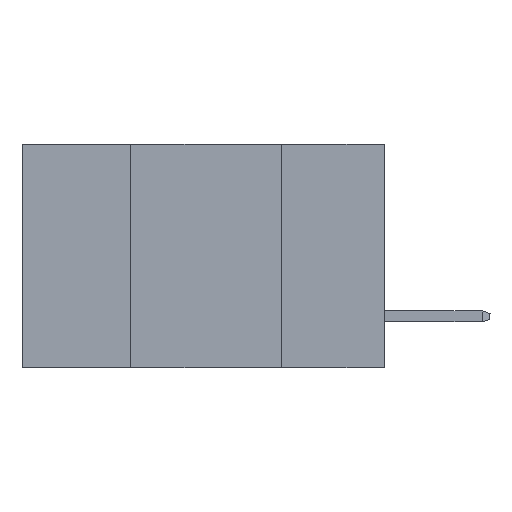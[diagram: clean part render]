
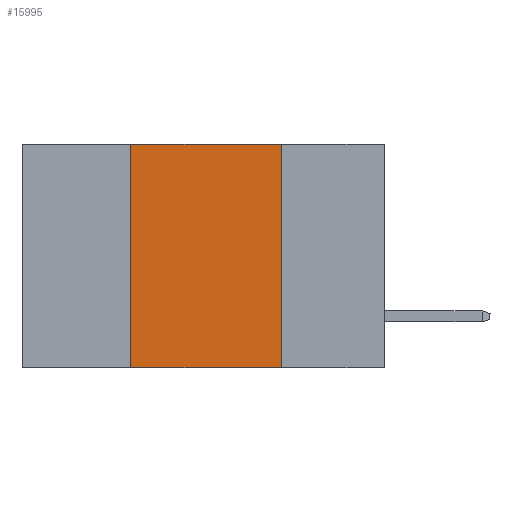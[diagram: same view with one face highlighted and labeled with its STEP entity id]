
A CAD part, left-side view. The second image highlights one B-rep face of the part: STEP entity #15995.
In plain terms, the highlighted planar face has unit normal (-1, 0, 0).
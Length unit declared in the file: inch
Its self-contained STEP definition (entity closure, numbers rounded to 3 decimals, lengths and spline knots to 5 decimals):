
#517 = CARTESIAN_POINT ( 'NONE',  ( 0., 0.42, -0.37 ) ) ;
#881 = CARTESIAN_POINT ( 'NONE',  ( 0., 0.42, 0. ) ) ;
#2649 = VERTEX_POINT ( 'NONE', #4060 ) ;
#3431 = PLANE ( 'NONE',  #14993 ) ;
#4060 = CARTESIAN_POINT ( 'NONE',  ( 0., 0.17, -0.37 ) ) ;
#5919 = VECTOR ( 'NONE', #8577, 39.37008 ) ;
#6310 = CARTESIAN_POINT ( 'NONE',  ( 0., 0.17, -0.37 ) ) ;
#6370 = DIRECTION ( 'NONE',  ( 0., 0., 1. ) ) ;
#7800 = EDGE_CURVE ( 'NONE', #10996, #2649, #8306, .T. ) ;
#7989 = LINE ( 'NONE', #12266, #12057 ) ;
#8306 = LINE ( 'NONE', #6310, #5919 ) ;
#8346 = VECTOR ( 'NONE', #24233, 39.37008 ) ;
#8577 = DIRECTION ( 'NONE',  ( 0., 0., -1. ) ) ;
#8600 = CARTESIAN_POINT ( 'NONE',  ( 0., 0.42, -0.37 ) ) ;
#8635 = EDGE_CURVE ( 'NONE', #16267, #10996, #7989, .T. ) ;
#8816 = ORIENTED_EDGE ( 'NONE', *, *, #8635, .F. ) ;
#10200 = CARTESIAN_POINT ( 'NONE',  ( 0., 0.6, -0.37 ) ) ;
#10996 = VERTEX_POINT ( 'NONE', #22782 ) ;
#12038 = EDGE_LOOP ( 'NONE', ( #16920, #8816, #14493, #23901 ) ) ;
#12057 = VECTOR ( 'NONE', #16145, 39.37008 ) ;
#12266 = CARTESIAN_POINT ( 'NONE',  ( 0., 0.6, 0. ) ) ;
#13305 = VECTOR ( 'NONE', #6370, 39.37008 ) ;
#14337 = LINE ( 'NONE', #10200, #8346 ) ;
#14414 = EDGE_CURVE ( 'NONE', #20551, #16267, #20670, .T. ) ;
#14493 = ORIENTED_EDGE ( 'NONE', *, *, #14414, .F. ) ;
#14495 = DIRECTION ( 'NONE',  ( 1., 0., 0. ) ) ;
#14993 = AXIS2_PLACEMENT_3D ( 'NONE', #24127, #14495, #22643 ) ;
#15995 = ADVANCED_FACE ( 'NONE', ( #22122 ), #3431, .F. ) ;
#16145 = DIRECTION ( 'NONE',  ( 0., -1., 0. ) ) ;
#16267 = VERTEX_POINT ( 'NONE', #881 ) ;
#16920 = ORIENTED_EDGE ( 'NONE', *, *, #7800, .F. ) ;
#20551 = VERTEX_POINT ( 'NONE', #8600 ) ;
#20670 = LINE ( 'NONE', #517, #13305 ) ;
#22122 = FACE_OUTER_BOUND ( 'NONE', #12038, .T. ) ;
#22643 = DIRECTION ( 'NONE',  ( 0., 0., -1. ) ) ;
#22678 = EDGE_CURVE ( 'NONE', #20551, #2649, #14337, .T. ) ;
#22782 = CARTESIAN_POINT ( 'NONE',  ( 0., 0.17, 0. ) ) ;
#23901 = ORIENTED_EDGE ( 'NONE', *, *, #22678, .T. ) ;
#24127 = CARTESIAN_POINT ( 'NONE',  ( 0., 0.6, 0. ) ) ;
#24233 = DIRECTION ( 'NONE',  ( 0., -1., 0. ) ) ;
